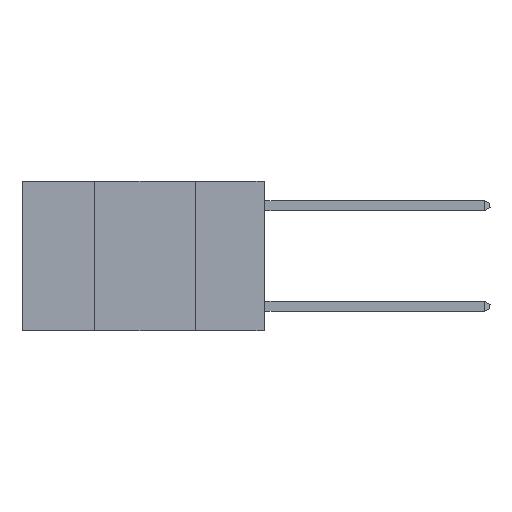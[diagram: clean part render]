
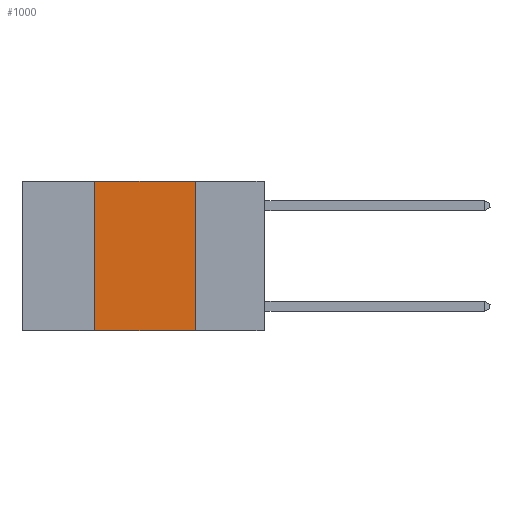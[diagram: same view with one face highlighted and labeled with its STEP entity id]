
A CAD part, left-side view. The second image highlights one B-rep face of the part: STEP entity #1000.
In plain terms, the highlighted planar face has unit normal (-1, 0, 0).
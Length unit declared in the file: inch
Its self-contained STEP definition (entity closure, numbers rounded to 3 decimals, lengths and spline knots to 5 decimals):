
#146 = VERTEX_POINT ( 'NONE', #8147 ) ;
#494 = DIRECTION ( 'NONE',  ( 0., -1., 0. ) ) ;
#684 = VECTOR ( 'NONE', #494, 39.37008 ) ;
#1000 = ADVANCED_FACE ( 'NONE', ( #11024 ), #16009, .F. ) ;
#1226 = VERTEX_POINT ( 'NONE', #2676 ) ;
#1748 = LINE ( 'NONE', #5200, #684 ) ;
#1832 = EDGE_CURVE ( 'NONE', #15454, #1226, #10882, .T. ) ;
#1880 = ORIENTED_EDGE ( 'NONE', *, *, #5128, .F. ) ;
#2676 = CARTESIAN_POINT ( 'NONE',  ( 0., 0.17, -0.37 ) ) ;
#2821 = CARTESIAN_POINT ( 'NONE',  ( 0., 0.42, 0. ) ) ;
#2845 = ORIENTED_EDGE ( 'NONE', *, *, #10517, .T. ) ;
#2931 = CARTESIAN_POINT ( 'NONE',  ( 0., 0.17, 0. ) ) ;
#3540 = LINE ( 'NONE', #4508, #9616 ) ;
#3878 = DIRECTION ( 'NONE',  ( 1., 0., 0. ) ) ;
#4508 = CARTESIAN_POINT ( 'NONE',  ( 0., 0.6, -0.37 ) ) ;
#5128 = EDGE_CURVE ( 'NONE', #11431, #15454, #1748, .T. ) ;
#5200 = CARTESIAN_POINT ( 'NONE',  ( 0., 0.6, 0. ) ) ;
#5441 = LINE ( 'NONE', #2821, #6370 ) ;
#5454 = CARTESIAN_POINT ( 'NONE',  ( 0., 0.6, 0. ) ) ;
#6370 = VECTOR ( 'NONE', #10518, 39.37008 ) ;
#6404 = CARTESIAN_POINT ( 'NONE',  ( 0., 0.17, 0. ) ) ;
#7562 = DIRECTION ( 'NONE',  ( 0., 0., -1. ) ) ;
#7929 = AXIS2_PLACEMENT_3D ( 'NONE', #5454, #3878, #7562 ) ;
#8147 = CARTESIAN_POINT ( 'NONE',  ( 0., 0.42, -0.37 ) ) ;
#8902 = DIRECTION ( 'NONE',  ( 0., 0., -1. ) ) ;
#9616 = VECTOR ( 'NONE', #15981, 39.37008 ) ;
#10100 = ORIENTED_EDGE ( 'NONE', *, *, #1832, .F. ) ;
#10517 = EDGE_CURVE ( 'NONE', #146, #1226, #3540, .T. ) ;
#10518 = DIRECTION ( 'NONE',  ( 0., 0., 1. ) ) ;
#10726 = EDGE_LOOP ( 'NONE', ( #10100, #1880, #10843, #2845 ) ) ;
#10843 = ORIENTED_EDGE ( 'NONE', *, *, #16008, .F. ) ;
#10882 = LINE ( 'NONE', #2931, #12145 ) ;
#11024 = FACE_OUTER_BOUND ( 'NONE', #10726, .T. ) ;
#11431 = VERTEX_POINT ( 'NONE', #13124 ) ;
#12145 = VECTOR ( 'NONE', #8902, 39.37008 ) ;
#13124 = CARTESIAN_POINT ( 'NONE',  ( 0., 0.42, 0. ) ) ;
#15454 = VERTEX_POINT ( 'NONE', #6404 ) ;
#15981 = DIRECTION ( 'NONE',  ( 0., -1., 0. ) ) ;
#16008 = EDGE_CURVE ( 'NONE', #146, #11431, #5441, .T. ) ;
#16009 = PLANE ( 'NONE',  #7929 ) ;
